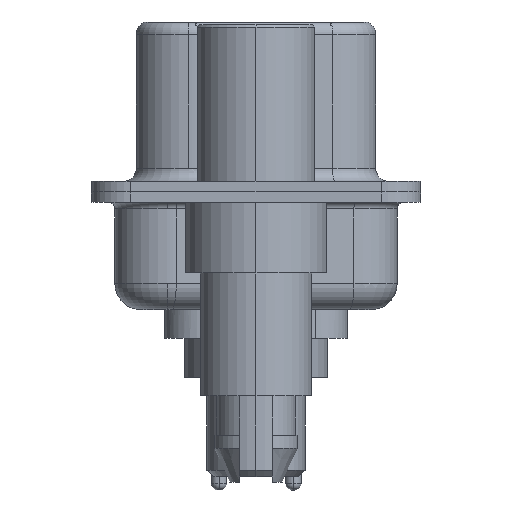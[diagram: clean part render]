
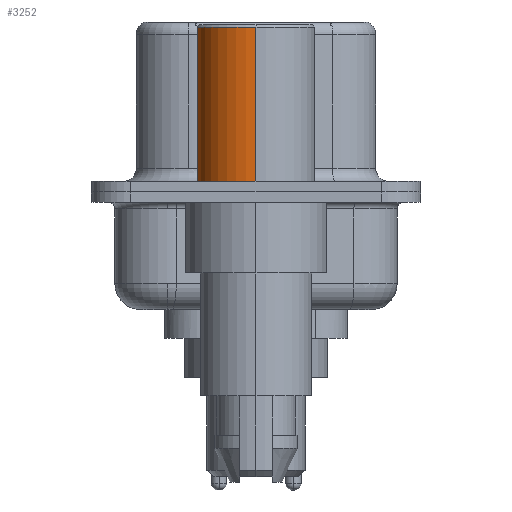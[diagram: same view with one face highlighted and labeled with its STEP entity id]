
A CAD part, left-side view. The second image highlights one B-rep face of the part: STEP entity #3252.
In plain terms, the highlighted cylindrical face has radius 2.25 mm (diameter 4.5 mm), a partial arc.
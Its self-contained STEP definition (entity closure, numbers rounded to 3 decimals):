
#715 = ORIENTED_EDGE ( 'NONE', *, *, #18024, .F. ) ;
#977 = DIRECTION ( 'NONE',  ( 1., 0., 0. ) ) ;
#2421 = CIRCLE ( 'NONE', #22242, 2.25 ) ;
#3252 = ADVANCED_FACE ( 'NONE', ( #9967 ), #4173, .T. ) ;
#4173 = CYLINDRICAL_SURFACE ( 'NONE', #21210, 2.25 ) ;
#5583 = VECTOR ( 'NONE', #21172, 1000. ) ;
#7042 = EDGE_CURVE ( 'NONE', #14348, #23750, #10778, .T. ) ;
#7060 = DIRECTION ( 'NONE',  ( 0., 0., 1. ) ) ;
#7412 = CARTESIAN_POINT ( 'NONE',  ( -2.25, 0., 0.4 ) ) ;
#8235 = AXIS2_PLACEMENT_3D ( 'NONE', #8700, #22141, #10683 ) ;
#8700 = CARTESIAN_POINT ( 'NONE',  ( 0., 0., 6.3 ) ) ;
#8993 = CARTESIAN_POINT ( 'NONE',  ( 0., 0., 0.4 ) ) ;
#9258 = EDGE_CURVE ( 'NONE', #14348, #10446, #2421, .T. ) ;
#9967 = FACE_OUTER_BOUND ( 'NONE', #22511, .T. ) ;
#10446 = VERTEX_POINT ( 'NONE', #7412 ) ;
#10683 = DIRECTION ( 'NONE',  ( 1., 0., 0. ) ) ;
#10778 = LINE ( 'NONE', #11637, #5583 ) ;
#10980 = DIRECTION ( 'NONE',  ( 1., 0., 0. ) ) ;
#11069 = CIRCLE ( 'NONE', #8235, 2.25 ) ;
#11637 = CARTESIAN_POINT ( 'NONE',  ( 2.25, 0., 0.581 ) ) ;
#12049 = ORIENTED_EDGE ( 'NONE', *, *, #9258, .T. ) ;
#12089 = EDGE_CURVE ( 'NONE', #10446, #12095, #24507, .T. ) ;
#12095 = VERTEX_POINT ( 'NONE', #21895 ) ;
#12315 = ORIENTED_EDGE ( 'NONE', *, *, #7042, .F. ) ;
#14344 = ORIENTED_EDGE ( 'NONE', *, *, #12089, .T. ) ;
#14348 = VERTEX_POINT ( 'NONE', #18733 ) ;
#18024 = EDGE_CURVE ( 'NONE', #23750, #12095, #11069, .T. ) ;
#18733 = CARTESIAN_POINT ( 'NONE',  ( 2.25, 0., 0.4 ) ) ;
#19548 = VECTOR ( 'NONE', #20038, 1000. ) ;
#20038 = DIRECTION ( 'NONE',  ( 0., 0., 1. ) ) ;
#21172 = DIRECTION ( 'NONE',  ( 0., 0., 1. ) ) ;
#21210 = AXIS2_PLACEMENT_3D ( 'NONE', #24031, #7060, #977 ) ;
#21740 = CARTESIAN_POINT ( 'NONE',  ( -2.25, 0., 0.581 ) ) ;
#21895 = CARTESIAN_POINT ( 'NONE',  ( -2.25, 0., 6.3 ) ) ;
#22141 = DIRECTION ( 'NONE',  ( 0., 0., 1. ) ) ;
#22242 = AXIS2_PLACEMENT_3D ( 'NONE', #8993, #22419, #10980 ) ;
#22419 = DIRECTION ( 'NONE',  ( 0., 0., 1. ) ) ;
#22511 = EDGE_LOOP ( 'NONE', ( #12049, #14344, #715, #12315 ) ) ;
#23750 = VERTEX_POINT ( 'NONE', #24838 ) ;
#24031 = CARTESIAN_POINT ( 'NONE',  ( 0., 0., 0.581 ) ) ;
#24507 = LINE ( 'NONE', #21740, #19548 ) ;
#24838 = CARTESIAN_POINT ( 'NONE',  ( 2.25, 0., 6.3 ) ) ;
